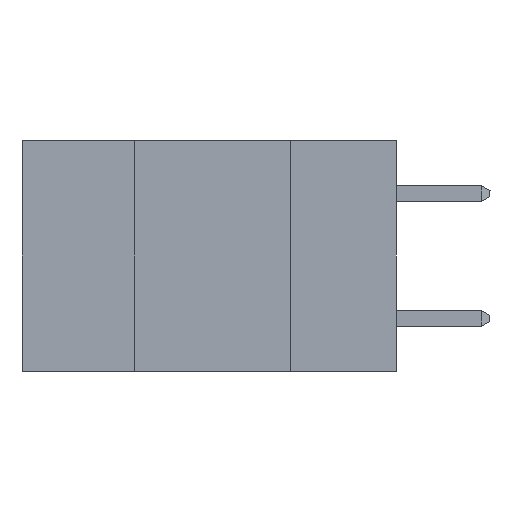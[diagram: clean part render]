
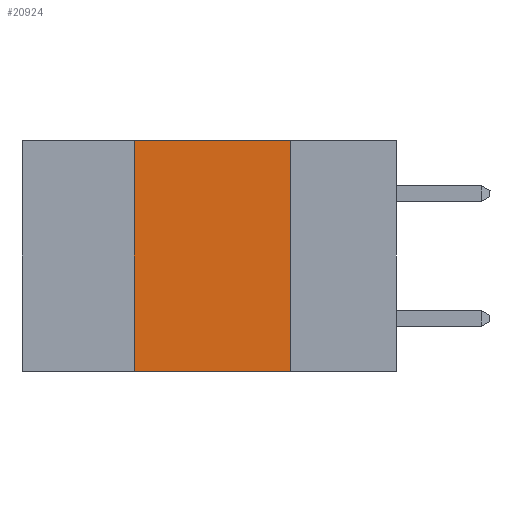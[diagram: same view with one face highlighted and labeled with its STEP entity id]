
A CAD part, left-side view. The second image highlights one B-rep face of the part: STEP entity #20924.
In plain terms, the highlighted planar face has unit normal (-1, 0, 0).
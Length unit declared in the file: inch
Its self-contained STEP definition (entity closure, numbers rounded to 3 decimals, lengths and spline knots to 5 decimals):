
#1395 = LINE ( 'NONE', #22173, #22643 ) ;
#1926 = ORIENTED_EDGE ( 'NONE', *, *, #5576, .F. ) ;
#2679 = DIRECTION ( 'NONE',  ( 0., 0., -1. ) ) ;
#2975 = CARTESIAN_POINT ( 'NONE',  ( 0., 0.17, -0.37 ) ) ;
#3470 = VERTEX_POINT ( 'NONE', #25469 ) ;
#4160 = EDGE_CURVE ( 'NONE', #4569, #14096, #1395, .T. ) ;
#4569 = VERTEX_POINT ( 'NONE', #8113 ) ;
#5321 = LINE ( 'NONE', #12039, #26531 ) ;
#5555 = LINE ( 'NONE', #2975, #26678 ) ;
#5576 = EDGE_CURVE ( 'NONE', #3470, #14096, #5555, .T. ) ;
#5992 = CARTESIAN_POINT ( 'NONE',  ( 0., 0.42, 0. ) ) ;
#6512 = CARTESIAN_POINT ( 'NONE',  ( 0., 0.17, -0.37 ) ) ;
#7280 = DIRECTION ( 'NONE',  ( 0., -1., 0. ) ) ;
#7575 = DIRECTION ( 'NONE',  ( 1., 0., 0. ) ) ;
#7866 = DIRECTION ( 'NONE',  ( 0., 0., 1. ) ) ;
#8058 = EDGE_CURVE ( 'NONE', #10382, #3470, #18756, .T. ) ;
#8113 = CARTESIAN_POINT ( 'NONE',  ( 0., 0.42, -0.37 ) ) ;
#9464 = AXIS2_PLACEMENT_3D ( 'NONE', #19839, #7575, #21894 ) ;
#10231 = EDGE_LOOP ( 'NONE', ( #1926, #12929, #19628, #26383 ) ) ;
#10382 = VERTEX_POINT ( 'NONE', #5992 ) ;
#12039 = CARTESIAN_POINT ( 'NONE',  ( 0., 0.42, -0.37 ) ) ;
#12929 = ORIENTED_EDGE ( 'NONE', *, *, #8058, .F. ) ;
#13854 = EDGE_CURVE ( 'NONE', #4569, #10382, #5321, .T. ) ;
#14096 = VERTEX_POINT ( 'NONE', #6512 ) ;
#15700 = PLANE ( 'NONE',  #9464 ) ;
#18756 = LINE ( 'NONE', #21585, #23587 ) ;
#19628 = ORIENTED_EDGE ( 'NONE', *, *, #13854, .F. ) ;
#19839 = CARTESIAN_POINT ( 'NONE',  ( 0., 0.6, 0. ) ) ;
#20924 = ADVANCED_FACE ( 'NONE', ( #22711 ), #15700, .F. ) ;
#21585 = CARTESIAN_POINT ( 'NONE',  ( 0., 0.6, 0. ) ) ;
#21894 = DIRECTION ( 'NONE',  ( 0., 0., -1. ) ) ;
#22173 = CARTESIAN_POINT ( 'NONE',  ( 0., 0.6, -0.37 ) ) ;
#22349 = DIRECTION ( 'NONE',  ( 0., -1., 0. ) ) ;
#22643 = VECTOR ( 'NONE', #22349, 39.37008 ) ;
#22711 = FACE_OUTER_BOUND ( 'NONE', #10231, .T. ) ;
#23587 = VECTOR ( 'NONE', #7280, 39.37008 ) ;
#25469 = CARTESIAN_POINT ( 'NONE',  ( 0., 0.17, 0. ) ) ;
#26383 = ORIENTED_EDGE ( 'NONE', *, *, #4160, .T. ) ;
#26531 = VECTOR ( 'NONE', #7866, 39.37008 ) ;
#26678 = VECTOR ( 'NONE', #2679, 39.37008 ) ;
